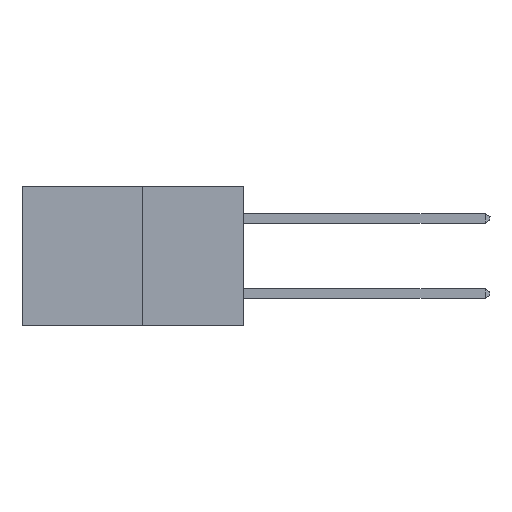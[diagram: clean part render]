
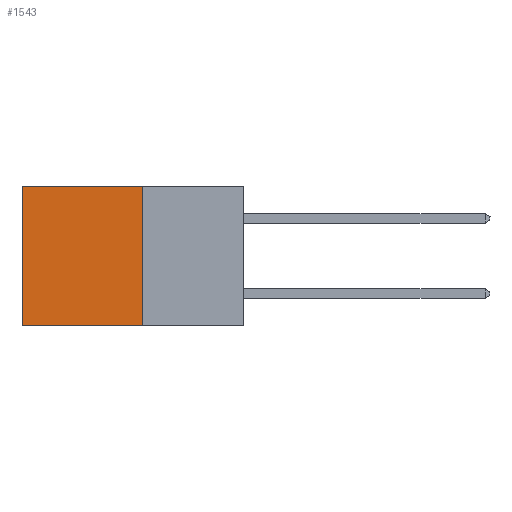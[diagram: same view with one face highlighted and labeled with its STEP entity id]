
A CAD part, left-side view. The second image highlights one B-rep face of the part: STEP entity #1543.
In plain terms, the highlighted planar face has unit normal (-1, 0, 0).
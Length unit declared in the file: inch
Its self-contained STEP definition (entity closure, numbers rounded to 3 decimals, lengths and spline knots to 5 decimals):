
#608 = ORIENTED_EDGE ( 'NONE', *, *, #1989, .F. ) ;
#1543 = ADVANCED_FACE ( 'NONE', ( #1879 ), #2580, .F. ) ;
#1581 = EDGE_CURVE ( 'NONE', #5049, #8990, #8997, .T. ) ;
#1830 = CARTESIAN_POINT ( 'NONE',  ( 0.277, 0.59, -0.37 ) ) ;
#1879 = FACE_OUTER_BOUND ( 'NONE', #2205, .T. ) ;
#1912 = CARTESIAN_POINT ( 'NONE',  ( 0.277, 0.27, 0. ) ) ;
#1989 = EDGE_CURVE ( 'NONE', #4805, #5049, #2081, .T. ) ;
#2067 = DIRECTION ( 'NONE',  ( 0., 1., 0. ) ) ;
#2081 = LINE ( 'NONE', #2132, #5632 ) ;
#2132 = CARTESIAN_POINT ( 'NONE',  ( 0.277, 0.27, -0.37 ) ) ;
#2205 = EDGE_LOOP ( 'NONE', ( #4235, #7891, #608, #4463 ) ) ;
#2580 = PLANE ( 'NONE',  #7303 ) ;
#2899 = DIRECTION ( 'NONE',  ( 0., 0., -1. ) ) ;
#3167 = CARTESIAN_POINT ( 'NONE',  ( 0.277, 0.59, -0.37 ) ) ;
#3793 = VECTOR ( 'NONE', #2067, 39.37008 ) ;
#4235 = ORIENTED_EDGE ( 'NONE', *, *, #6133, .T. ) ;
#4463 = ORIENTED_EDGE ( 'NONE', *, *, #5794, .T. ) ;
#4805 = VERTEX_POINT ( 'NONE', #1912 ) ;
#5049 = VERTEX_POINT ( 'NONE', #6026 ) ;
#5627 = CARTESIAN_POINT ( 'NONE',  ( 0.277, 0.27, -0.37 ) ) ;
#5632 = VECTOR ( 'NONE', #2899, 39.37008 ) ;
#5794 = EDGE_CURVE ( 'NONE', #4805, #8001, #7939, .T. ) ;
#6026 = CARTESIAN_POINT ( 'NONE',  ( 0.277, 0.27, -0.37 ) ) ;
#6125 = VECTOR ( 'NONE', #7698, 39.37008 ) ;
#6133 = EDGE_CURVE ( 'NONE', #8001, #8990, #8746, .T. ) ;
#7029 = CARTESIAN_POINT ( 'NONE',  ( 0.277, 0.27, 0. ) ) ;
#7211 = CARTESIAN_POINT ( 'NONE',  ( 0.277, 0.27, -0.37 ) ) ;
#7303 = AXIS2_PLACEMENT_3D ( 'NONE', #7211, #8628, #8428 ) ;
#7618 = VECTOR ( 'NONE', #8752, 39.37008 ) ;
#7698 = DIRECTION ( 'NONE',  ( 0., 1., 0. ) ) ;
#7891 = ORIENTED_EDGE ( 'NONE', *, *, #1581, .F. ) ;
#7939 = LINE ( 'NONE', #7029, #6125 ) ;
#8001 = VERTEX_POINT ( 'NONE', #8190 ) ;
#8190 = CARTESIAN_POINT ( 'NONE',  ( 0.277, 0.59, 0. ) ) ;
#8428 = DIRECTION ( 'NONE',  ( 0., 0., -1. ) ) ;
#8628 = DIRECTION ( 'NONE',  ( 1., 0., 0. ) ) ;
#8746 = LINE ( 'NONE', #1830, #7618 ) ;
#8752 = DIRECTION ( 'NONE',  ( 0., 0., -1. ) ) ;
#8990 = VERTEX_POINT ( 'NONE', #3167 ) ;
#8997 = LINE ( 'NONE', #5627, #3793 ) ;
